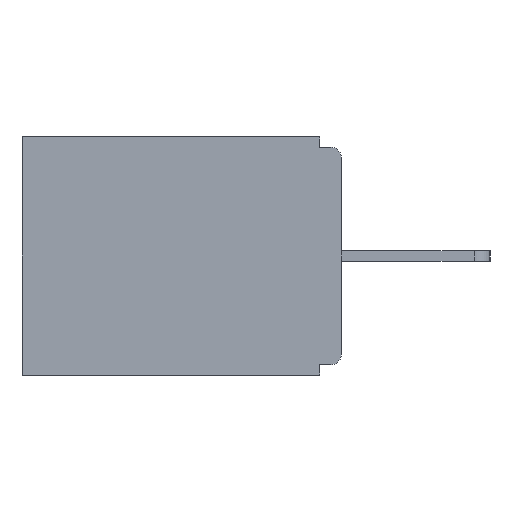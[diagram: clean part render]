
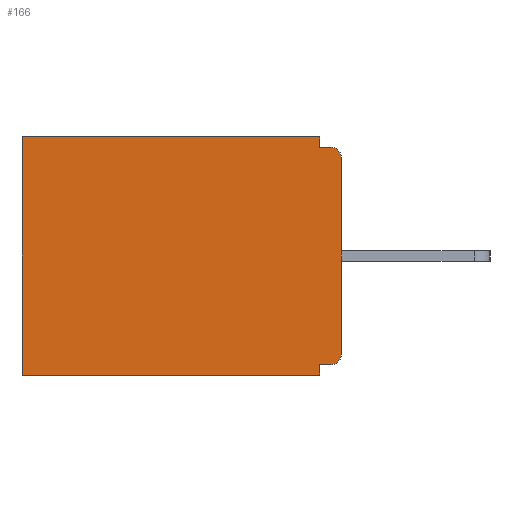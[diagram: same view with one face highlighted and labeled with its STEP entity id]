
A CAD part, left-side view. The second image highlights one B-rep face of the part: STEP entity #166.
In plain terms, the highlighted planar face has unit normal (-1, 0, 0).
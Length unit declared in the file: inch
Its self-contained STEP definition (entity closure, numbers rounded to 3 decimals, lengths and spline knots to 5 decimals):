
#6 = CARTESIAN_POINT ( 'NONE',  ( 0.298, 0.031, -0.343 ) ) ;
#50 = VERTEX_POINT ( 'NONE', #7254 ) ;
#166 = ADVANCED_FACE ( 'NONE', ( #7177 ), #4141, .F. ) ;
#235 = VERTEX_POINT ( 'NONE', #649 ) ;
#294 = ORIENTED_EDGE ( 'NONE', *, *, #4842, .T. ) ;
#333 = CARTESIAN_POINT ( 'NONE',  ( 0.298, 0., -0.343 ) ) ;
#407 = CARTESIAN_POINT ( 'NONE',  ( 0.298, 0.015, -0.328 ) ) ;
#649 = CARTESIAN_POINT ( 'NONE',  ( 0.298, 0.031, -0.015 ) ) ;
#837 = ORIENTED_EDGE ( 'NONE', *, *, #4408, .T. ) ;
#842 = EDGE_CURVE ( 'NONE', #4878, #50, #8915, .T. ) ;
#900 = ORIENTED_EDGE ( 'NONE', *, *, #1675, .F. ) ;
#987 = DIRECTION ( 'NONE',  ( 0., 0., -1. ) ) ;
#999 = VERTEX_POINT ( 'NONE', #1694 ) ;
#1022 = LINE ( 'NONE', #11315, #3300 ) ;
#1218 = ORIENTED_EDGE ( 'NONE', *, *, #9082, .F. ) ;
#1248 = DIRECTION ( 'NONE',  ( 0., 0., -1. ) ) ;
#1288 = DIRECTION ( 'NONE',  ( 1., 0., 0. ) ) ;
#1504 = EDGE_CURVE ( 'NONE', #4866, #9431, #10813, .T. ) ;
#1565 = DIRECTION ( 'NONE',  ( 0., 0., -1. ) ) ;
#1600 = VECTOR ( 'NONE', #1248, 39.37008 ) ;
#1675 = EDGE_CURVE ( 'NONE', #999, #235, #1022, .T. ) ;
#1694 = CARTESIAN_POINT ( 'NONE',  ( 0.298, 0.031, 0. ) ) ;
#1874 = EDGE_CURVE ( 'NONE', #10117, #50, #6555, .T. ) ;
#2113 = DIRECTION ( 'NONE',  ( 0., 0., -1. ) ) ;
#2318 = CARTESIAN_POINT ( 'NONE',  ( 0.298, 0., -0.03 ) ) ;
#2481 = AXIS2_PLACEMENT_3D ( 'NONE', #11046, #1288, #1565 ) ;
#2522 = EDGE_CURVE ( 'NONE', #9431, #10117, #6536, .T. ) ;
#2646 = CARTESIAN_POINT ( 'NONE',  ( 0.298, 0.46, 0. ) ) ;
#2765 = CARTESIAN_POINT ( 'NONE',  ( 0.298, 0.46, 0. ) ) ;
#2766 = LINE ( 'NONE', #11248, #11366 ) ;
#2954 = CARTESIAN_POINT ( 'NONE',  ( 0.298, 0.031, -0.343 ) ) ;
#3300 = VECTOR ( 'NONE', #8789, 39.37008 ) ;
#3577 = EDGE_CURVE ( 'NONE', #235, #8549, #2766, .T. ) ;
#3643 = DIRECTION ( 'NONE',  ( -1., 0., 0. ) ) ;
#3657 = CARTESIAN_POINT ( 'NONE',  ( 0.298, 0.015, -0.313 ) ) ;
#3958 = DIRECTION ( 'NONE',  ( 0., 0., -1. ) ) ;
#4042 = EDGE_CURVE ( 'NONE', #4866, #7579, #8228, .T. ) ;
#4141 = PLANE ( 'NONE',  #2481 ) ;
#4253 = CARTESIAN_POINT ( 'NONE',  ( 0.298, 0.031, -0.328 ) ) ;
#4378 = VECTOR ( 'NONE', #10616, 39.37008 ) ;
#4408 = EDGE_CURVE ( 'NONE', #999, #4878, #10848, .T. ) ;
#4557 = EDGE_LOOP ( 'NONE', ( #294, #5605, #900, #837, #5871, #5929, #10523, #10309, #10784, #1218 ) ) ;
#4842 = EDGE_CURVE ( 'NONE', #9512, #8549, #11100, .T. ) ;
#4866 = VERTEX_POINT ( 'NONE', #407 ) ;
#4878 = VERTEX_POINT ( 'NONE', #2646 ) ;
#4895 = CARTESIAN_POINT ( 'NONE',  ( 0.298, 0., 0. ) ) ;
#5304 = CARTESIAN_POINT ( 'NONE',  ( 0.298, 0., -0.313 ) ) ;
#5605 = ORIENTED_EDGE ( 'NONE', *, *, #3577, .F. ) ;
#5871 = ORIENTED_EDGE ( 'NONE', *, *, #842, .T. ) ;
#5929 = ORIENTED_EDGE ( 'NONE', *, *, #1874, .F. ) ;
#6257 = CARTESIAN_POINT ( 'NONE',  ( 0.298, 0., 0. ) ) ;
#6379 = VECTOR ( 'NONE', #3958, 39.37008 ) ;
#6536 = LINE ( 'NONE', #6, #1600 ) ;
#6555 = LINE ( 'NONE', #333, #10917 ) ;
#7177 = FACE_OUTER_BOUND ( 'NONE', #4557, .T. ) ;
#7254 = CARTESIAN_POINT ( 'NONE',  ( 0.298, 0.46, -0.343 ) ) ;
#7494 = LINE ( 'NONE', #4895, #6379 ) ;
#7579 = VERTEX_POINT ( 'NONE', #5304 ) ;
#7640 = CARTESIAN_POINT ( 'NONE',  ( 0.298, 0.015, -0.03 ) ) ;
#7792 = DIRECTION ( 'NONE',  ( 0., 1., 0. ) ) ;
#7954 = CARTESIAN_POINT ( 'NONE',  ( 0.298, 0.015, -0.015 ) ) ;
#8228 = CIRCLE ( 'NONE', #9062, 0.015 ) ;
#8379 = CARTESIAN_POINT ( 'NONE',  ( 0.298, 0., -0.328 ) ) ;
#8483 = AXIS2_PLACEMENT_3D ( 'NONE', #7640, #11346, #987 ) ;
#8498 = DIRECTION ( 'NONE',  ( 0., 1., 0. ) ) ;
#8549 = VERTEX_POINT ( 'NONE', #7954 ) ;
#8789 = DIRECTION ( 'NONE',  ( 0., 0., -1. ) ) ;
#8915 = LINE ( 'NONE', #2765, #4378 ) ;
#9062 = AXIS2_PLACEMENT_3D ( 'NONE', #3657, #3643, #2113 ) ;
#9082 = EDGE_CURVE ( 'NONE', #9512, #7579, #7494, .T. ) ;
#9431 = VERTEX_POINT ( 'NONE', #4253 ) ;
#9512 = VERTEX_POINT ( 'NONE', #2318 ) ;
#10117 = VERTEX_POINT ( 'NONE', #2954 ) ;
#10309 = ORIENTED_EDGE ( 'NONE', *, *, #1504, .F. ) ;
#10523 = ORIENTED_EDGE ( 'NONE', *, *, #2522, .F. ) ;
#10616 = DIRECTION ( 'NONE',  ( 0., 0., -1. ) ) ;
#10771 = DIRECTION ( 'NONE',  ( 0., 1., 0. ) ) ;
#10784 = ORIENTED_EDGE ( 'NONE', *, *, #4042, .T. ) ;
#10813 = LINE ( 'NONE', #8379, #11063 ) ;
#10848 = LINE ( 'NONE', #6257, #11111 ) ;
#10917 = VECTOR ( 'NONE', #10771, 39.37008 ) ;
#11046 = CARTESIAN_POINT ( 'NONE',  ( 0.298, 0., 0. ) ) ;
#11063 = VECTOR ( 'NONE', #8498, 39.37008 ) ;
#11100 = CIRCLE ( 'NONE', #8483, 0.015 ) ;
#11111 = VECTOR ( 'NONE', #7792, 39.37008 ) ;
#11248 = CARTESIAN_POINT ( 'NONE',  ( 0.298, 0., -0.015 ) ) ;
#11283 = DIRECTION ( 'NONE',  ( 0., -1., 0. ) ) ;
#11315 = CARTESIAN_POINT ( 'NONE',  ( 0.298, 0.031, -0.343 ) ) ;
#11346 = DIRECTION ( 'NONE',  ( -1., 0., 0. ) ) ;
#11366 = VECTOR ( 'NONE', #11283, 39.37008 ) ;
